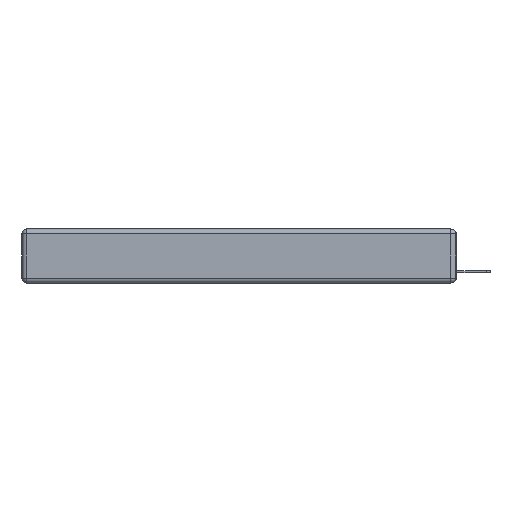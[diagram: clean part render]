
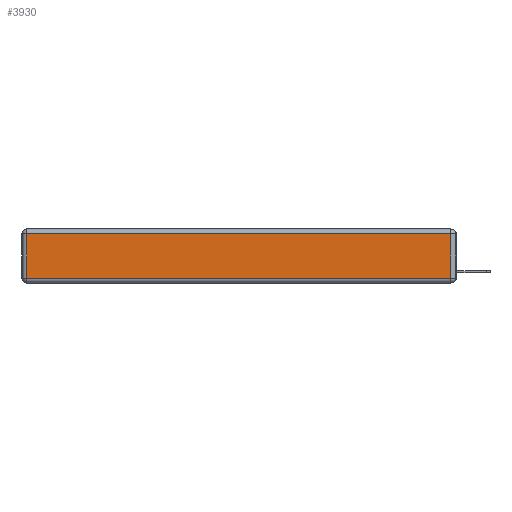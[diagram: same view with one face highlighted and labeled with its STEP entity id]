
A CAD part, left-side view. The second image highlights one B-rep face of the part: STEP entity #3930.
In plain terms, the highlighted planar face has unit normal (-1, 0, 0).
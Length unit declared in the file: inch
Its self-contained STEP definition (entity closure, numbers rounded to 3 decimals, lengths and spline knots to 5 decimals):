
#448 = PLANE ( 'NONE',  #3001 ) ;
#855 = DIRECTION ( 'NONE',  ( 0., 0., -1. ) ) ;
#1014 = VECTOR ( 'NONE', #9831, 39.37008 ) ;
#1135 = EDGE_CURVE ( 'NONE', #14824, #12797, #15234, .T. ) ;
#1864 = EDGE_LOOP ( 'NONE', ( #18033, #10237, #9856, #9449 ) ) ;
#2524 = EDGE_CURVE ( 'NONE', #5462, #15427, #18508, .T. ) ;
#2719 = CARTESIAN_POINT ( 'NONE',  ( 0., 2.72, -0.313 ) ) ;
#3001 = AXIS2_PLACEMENT_3D ( 'NONE', #12117, #10600, #17989 ) ;
#3930 = ADVANCED_FACE ( 'NONE', ( #7609 ), #448, .T. ) ;
#4673 = DIRECTION ( 'NONE',  ( 0., 0., 1. ) ) ;
#5351 = CARTESIAN_POINT ( 'NONE',  ( 0., 0.03, -0.343 ) ) ;
#5462 = VERTEX_POINT ( 'NONE', #14790 ) ;
#7609 = FACE_OUTER_BOUND ( 'NONE', #1864, .T. ) ;
#7892 = CARTESIAN_POINT ( 'NONE',  ( 0., 0., -0.313 ) ) ;
#8504 = VECTOR ( 'NONE', #4673, 39.37008 ) ;
#8725 = LINE ( 'NONE', #17101, #12071 ) ;
#9449 = ORIENTED_EDGE ( 'NONE', *, *, #1135, .T. ) ;
#9542 = LINE ( 'NONE', #7892, #1014 ) ;
#9745 = VECTOR ( 'NONE', #855, 39.37008 ) ;
#9831 = DIRECTION ( 'NONE',  ( 0., -1., 0. ) ) ;
#9856 = ORIENTED_EDGE ( 'NONE', *, *, #18770, .T. ) ;
#10237 = ORIENTED_EDGE ( 'NONE', *, *, #2524, .T. ) ;
#10600 = DIRECTION ( 'NONE',  ( -1., 0., 0. ) ) ;
#10634 = CARTESIAN_POINT ( 'NONE',  ( 0., 2.72, -0.343 ) ) ;
#12071 = VECTOR ( 'NONE', #15751, 39.37008 ) ;
#12117 = CARTESIAN_POINT ( 'NONE',  ( 0., 0., -0.343 ) ) ;
#12663 = CARTESIAN_POINT ( 'NONE',  ( 0., 0.03, -0.03 ) ) ;
#12797 = VERTEX_POINT ( 'NONE', #2719 ) ;
#14269 = CARTESIAN_POINT ( 'NONE',  ( 0., 2.72, -0.03 ) ) ;
#14790 = CARTESIAN_POINT ( 'NONE',  ( 0., 0.03, -0.313 ) ) ;
#14824 = VERTEX_POINT ( 'NONE', #14269 ) ;
#15234 = LINE ( 'NONE', #10634, #9745 ) ;
#15427 = VERTEX_POINT ( 'NONE', #12663 ) ;
#15751 = DIRECTION ( 'NONE',  ( 0., 1., 0. ) ) ;
#16474 = EDGE_CURVE ( 'NONE', #12797, #5462, #9542, .T. ) ;
#17101 = CARTESIAN_POINT ( 'NONE',  ( 0., 2.75, -0.03 ) ) ;
#17989 = DIRECTION ( 'NONE',  ( 0., 0., 1. ) ) ;
#18033 = ORIENTED_EDGE ( 'NONE', *, *, #16474, .T. ) ;
#18508 = LINE ( 'NONE', #5351, #8504 ) ;
#18770 = EDGE_CURVE ( 'NONE', #15427, #14824, #8725, .T. ) ;
